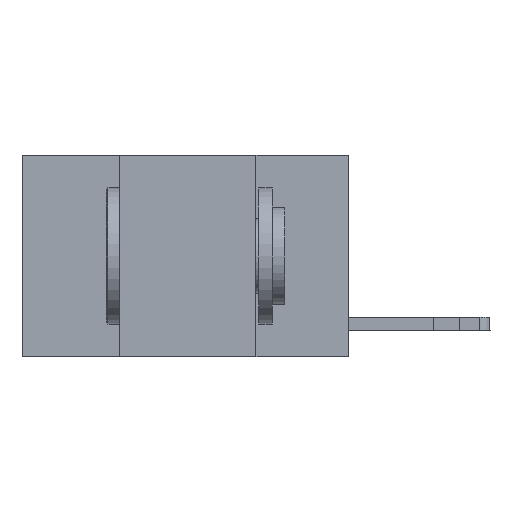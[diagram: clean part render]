
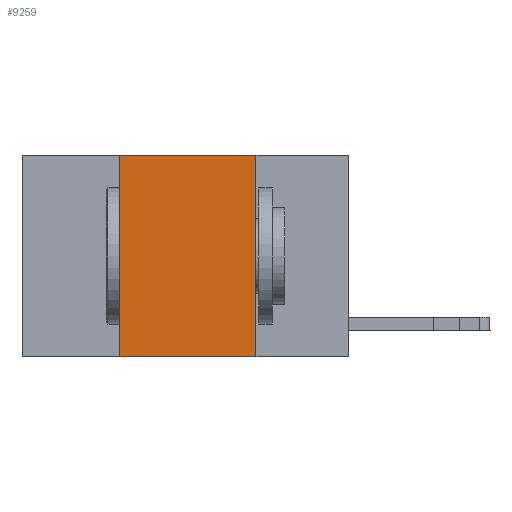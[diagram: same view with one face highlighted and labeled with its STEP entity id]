
A CAD part, left-side view. The second image highlights one B-rep face of the part: STEP entity #9259.
In plain terms, the highlighted planar face has unit normal (-1, 0, 0).
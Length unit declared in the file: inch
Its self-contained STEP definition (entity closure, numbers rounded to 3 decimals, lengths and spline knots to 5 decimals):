
#381 = CARTESIAN_POINT ( 'NONE',  ( 0., 0.6, 0. ) ) ;
#1609 = VERTEX_POINT ( 'NONE', #10658 ) ;
#1728 = CARTESIAN_POINT ( 'NONE',  ( 0., 0.6, -0.37 ) ) ;
#2133 = ORIENTED_EDGE ( 'NONE', *, *, #2377, .F. ) ;
#2159 = ORIENTED_EDGE ( 'NONE', *, *, #7593, .F. ) ;
#2377 = EDGE_CURVE ( 'NONE', #1609, #3122, #23150, .T. ) ;
#2937 = ORIENTED_EDGE ( 'NONE', *, *, #12519, .F. ) ;
#3122 = VERTEX_POINT ( 'NONE', #4560 ) ;
#3781 = VECTOR ( 'NONE', #4781, 39.37008 ) ;
#4560 = CARTESIAN_POINT ( 'NONE',  ( 0., 0.17, 0. ) ) ;
#4779 = AXIS2_PLACEMENT_3D ( 'NONE', #22456, #20333, #20208 ) ;
#4781 = DIRECTION ( 'NONE',  ( 0., 0., 1. ) ) ;
#5104 = LINE ( 'NONE', #21800, #24282 ) ;
#6363 = LINE ( 'NONE', #11954, #3781 ) ;
#7221 = LINE ( 'NONE', #1728, #10978 ) ;
#7495 = VERTEX_POINT ( 'NONE', #23431 ) ;
#7593 = EDGE_CURVE ( 'NONE', #3122, #8506, #5104, .T. ) ;
#8506 = VERTEX_POINT ( 'NONE', #16837 ) ;
#9259 = ADVANCED_FACE ( 'NONE', ( #12664 ), #18570, .F. ) ;
#10053 = DIRECTION ( 'NONE',  ( 0., -1., 0. ) ) ;
#10592 = DIRECTION ( 'NONE',  ( 0., 0., -1. ) ) ;
#10658 = CARTESIAN_POINT ( 'NONE',  ( 0., 0.42, 0. ) ) ;
#10978 = VECTOR ( 'NONE', #14663, 39.37008 ) ;
#11954 = CARTESIAN_POINT ( 'NONE',  ( 0., 0.42, 0. ) ) ;
#12519 = EDGE_CURVE ( 'NONE', #7495, #1609, #6363, .T. ) ;
#12664 = FACE_OUTER_BOUND ( 'NONE', #20095, .T. ) ;
#14663 = DIRECTION ( 'NONE',  ( 0., -1., 0. ) ) ;
#16837 = CARTESIAN_POINT ( 'NONE',  ( 0., 0.17, -0.37 ) ) ;
#17081 = EDGE_CURVE ( 'NONE', #7495, #8506, #7221, .T. ) ;
#17362 = ORIENTED_EDGE ( 'NONE', *, *, #17081, .T. ) ;
#18570 = PLANE ( 'NONE',  #4779 ) ;
#20095 = EDGE_LOOP ( 'NONE', ( #2159, #2133, #2937, #17362 ) ) ;
#20208 = DIRECTION ( 'NONE',  ( 0., 0., -1. ) ) ;
#20333 = DIRECTION ( 'NONE',  ( 1., 0., 0. ) ) ;
#21800 = CARTESIAN_POINT ( 'NONE',  ( 0., 0.17, 0. ) ) ;
#22456 = CARTESIAN_POINT ( 'NONE',  ( 0., 0.6, 0. ) ) ;
#23150 = LINE ( 'NONE', #381, #24158 ) ;
#23431 = CARTESIAN_POINT ( 'NONE',  ( 0., 0.42, -0.37 ) ) ;
#24158 = VECTOR ( 'NONE', #10053, 39.37008 ) ;
#24282 = VECTOR ( 'NONE', #10592, 39.37008 ) ;
